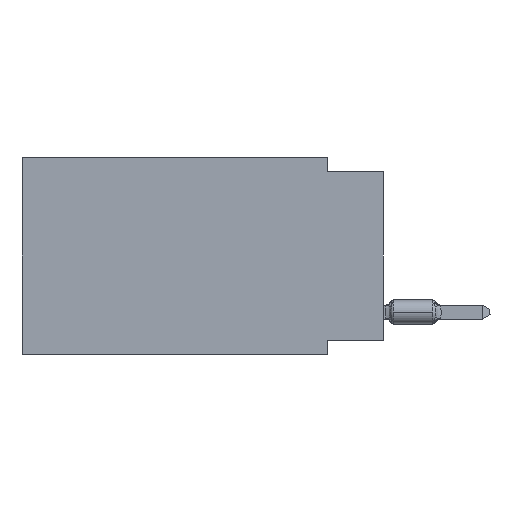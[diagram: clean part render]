
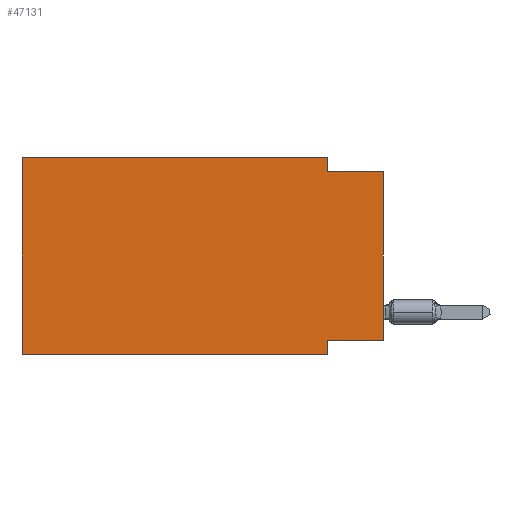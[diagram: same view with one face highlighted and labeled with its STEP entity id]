
A CAD part, left-side view. The second image highlights one B-rep face of the part: STEP entity #47131.
In plain terms, the highlighted planar face has unit normal (-1, 0, 0).
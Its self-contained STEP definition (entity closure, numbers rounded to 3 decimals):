
#1309 = DIRECTION ( 'NONE',  ( 1., 0., 0. ) ) ;
#1777 = CARTESIAN_POINT ( 'NONE',  ( 0., 0., -8.255 ) ) ;
#2277 = EDGE_CURVE ( 'NONE', #19719, #46402, #3701, .T. ) ;
#3169 = EDGE_CURVE ( 'NONE', #41703, #21737, #38719, .T. ) ;
#3701 = LINE ( 'NONE', #64328, #13161 ) ;
#5359 = CARTESIAN_POINT ( 'NONE',  ( 0., 0., -8.255 ) ) ;
#7469 = CARTESIAN_POINT ( 'NONE',  ( 0., 16.383, -8.89 ) ) ;
#10627 = ORIENTED_EDGE ( 'NONE', *, *, #51171, .F. ) ;
#11338 = EDGE_CURVE ( 'NONE', #39457, #46402, #57641, .T. ) ;
#13161 = VECTOR ( 'NONE', #29284, 1000. ) ;
#16142 = VERTEX_POINT ( 'NONE', #43220 ) ;
#17768 = AXIS2_PLACEMENT_3D ( 'NONE', #46247, #1309, #61275 ) ;
#19085 = VECTOR ( 'NONE', #40638, 1000. ) ;
#19719 = VERTEX_POINT ( 'NONE', #48929 ) ;
#20637 = CARTESIAN_POINT ( 'NONE',  ( 0., 16.383, 0. ) ) ;
#20757 = VECTOR ( 'NONE', #25362, 1000. ) ;
#21737 = VERTEX_POINT ( 'NONE', #36847 ) ;
#21807 = DIRECTION ( 'NONE',  ( 0., 1., 0. ) ) ;
#25333 = CARTESIAN_POINT ( 'NONE',  ( 0., 2.54, 0. ) ) ;
#25362 = DIRECTION ( 'NONE',  ( 0., 0., 1. ) ) ;
#25559 = LINE ( 'NONE', #20637, #19085 ) ;
#26122 = ORIENTED_EDGE ( 'NONE', *, *, #40337, .F. ) ;
#26151 = CARTESIAN_POINT ( 'NONE',  ( 0., 2.54, 0. ) ) ;
#26232 = PLANE ( 'NONE',  #17768 ) ;
#26625 = EDGE_LOOP ( 'NONE', ( #31009, #51184, #32943, #10627, #38491, #30849, #37838, #26122 ) ) ;
#27918 = VECTOR ( 'NONE', #37426, 1000. ) ;
#28170 = VECTOR ( 'NONE', #42580, 1000. ) ;
#29284 = DIRECTION ( 'NONE',  ( 0., 0., -1. ) ) ;
#29315 = EDGE_CURVE ( 'NONE', #61998, #21737, #34481, .T. ) ;
#30170 = EDGE_CURVE ( 'NONE', #39457, #16142, #30262, .T. ) ;
#30262 = LINE ( 'NONE', #41405, #20757 ) ;
#30520 = CARTESIAN_POINT ( 'NONE',  ( 0., 0., -0.635 ) ) ;
#30849 = ORIENTED_EDGE ( 'NONE', *, *, #11338, .T. ) ;
#31009 = ORIENTED_EDGE ( 'NONE', *, *, #3169, .T. ) ;
#32221 = VECTOR ( 'NONE', #60635, 1000. ) ;
#32943 = ORIENTED_EDGE ( 'NONE', *, *, #47605, .F. ) ;
#34481 = LINE ( 'NONE', #30520, #32221 ) ;
#36294 = CARTESIAN_POINT ( 'NONE',  ( 0., 2.54, -0.635 ) ) ;
#36847 = CARTESIAN_POINT ( 'NONE',  ( 0., 0., -0.635 ) ) ;
#37426 = DIRECTION ( 'NONE',  ( 0., 0., 1. ) ) ;
#37838 = ORIENTED_EDGE ( 'NONE', *, *, #2277, .F. ) ;
#38491 = ORIENTED_EDGE ( 'NONE', *, *, #30170, .F. ) ;
#38719 = LINE ( 'NONE', #48569, #27918 ) ;
#39457 = VERTEX_POINT ( 'NONE', #63566 ) ;
#40337 = EDGE_CURVE ( 'NONE', #41703, #19719, #46727, .T. ) ;
#40638 = DIRECTION ( 'NONE',  ( 0., -1., 0. ) ) ;
#41405 = CARTESIAN_POINT ( 'NONE',  ( 0., 16.383, 0. ) ) ;
#41703 = VERTEX_POINT ( 'NONE', #5359 ) ;
#42580 = DIRECTION ( 'NONE',  ( 0., -1., 0. ) ) ;
#43220 = CARTESIAN_POINT ( 'NONE',  ( 0., 16.383, 0. ) ) ;
#44039 = VECTOR ( 'NONE', #44991, 1000. ) ;
#44991 = DIRECTION ( 'NONE',  ( 0., 0., -1. ) ) ;
#46247 = CARTESIAN_POINT ( 'NONE',  ( 0., 16.383, 0. ) ) ;
#46402 = VERTEX_POINT ( 'NONE', #58151 ) ;
#46727 = LINE ( 'NONE', #1777, #47067 ) ;
#47067 = VECTOR ( 'NONE', #21807, 1000. ) ;
#47131 = ADVANCED_FACE ( 'NONE', ( #51125 ), #26232, .F. ) ;
#47605 = EDGE_CURVE ( 'NONE', #64350, #61998, #60054, .T. ) ;
#48569 = CARTESIAN_POINT ( 'NONE',  ( 0., 0., 0. ) ) ;
#48929 = CARTESIAN_POINT ( 'NONE',  ( 0., 2.54, -8.255 ) ) ;
#51125 = FACE_OUTER_BOUND ( 'NONE', #26625, .T. ) ;
#51171 = EDGE_CURVE ( 'NONE', #16142, #64350, #25559, .T. ) ;
#51184 = ORIENTED_EDGE ( 'NONE', *, *, #29315, .F. ) ;
#57641 = LINE ( 'NONE', #7469, #28170 ) ;
#58151 = CARTESIAN_POINT ( 'NONE',  ( 0., 2.54, -8.89 ) ) ;
#60054 = LINE ( 'NONE', #25333, #44039 ) ;
#60635 = DIRECTION ( 'NONE',  ( 0., -1., 0. ) ) ;
#61275 = DIRECTION ( 'NONE',  ( 0., 0., -1. ) ) ;
#61998 = VERTEX_POINT ( 'NONE', #36294 ) ;
#63566 = CARTESIAN_POINT ( 'NONE',  ( 0., 16.383, -8.89 ) ) ;
#64328 = CARTESIAN_POINT ( 'NONE',  ( 0., 2.54, -8.89 ) ) ;
#64350 = VERTEX_POINT ( 'NONE', #26151 ) ;
